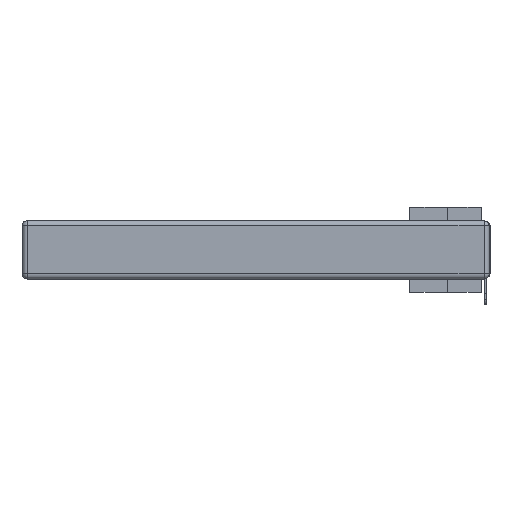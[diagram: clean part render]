
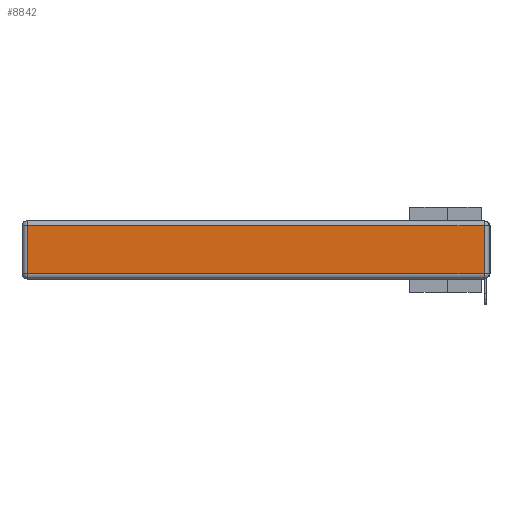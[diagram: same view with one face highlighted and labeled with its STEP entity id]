
A CAD part, left-side view. The second image highlights one B-rep face of the part: STEP entity #8842.
In plain terms, the highlighted planar face has unit normal (-1, 0, 0).
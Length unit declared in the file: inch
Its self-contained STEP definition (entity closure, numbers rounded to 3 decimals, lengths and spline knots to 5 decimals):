
#875 = CARTESIAN_POINT ( 'NONE',  ( 0., 2.75, -0.03 ) ) ;
#2345 = CARTESIAN_POINT ( 'NONE',  ( 0., 0.03, -0.03 ) ) ;
#2662 = DIRECTION ( 'NONE',  ( -1., 0., 0. ) ) ;
#2829 = CARTESIAN_POINT ( 'NONE',  ( 0., 0., -0.343 ) ) ;
#3519 = DIRECTION ( 'NONE',  ( 0., 1., 0. ) ) ;
#4431 = CARTESIAN_POINT ( 'NONE',  ( 0., 2.72, -0.343 ) ) ;
#6391 = EDGE_CURVE ( 'NONE', #31408, #27377, #11120, .T. ) ;
#7058 = ORIENTED_EDGE ( 'NONE', *, *, #6391, .T. ) ;
#8842 = ADVANCED_FACE ( 'NONE', ( #15121 ), #13142, .T. ) ;
#10361 = LINE ( 'NONE', #22984, #17152 ) ;
#10749 = VERTEX_POINT ( 'NONE', #23741 ) ;
#11120 = LINE ( 'NONE', #23893, #20728 ) ;
#11414 = EDGE_LOOP ( 'NONE', ( #19483, #7058, #20182, #12416 ) ) ;
#11934 = DIRECTION ( 'NONE',  ( 0., 0., -1. ) ) ;
#12416 = ORIENTED_EDGE ( 'NONE', *, *, #16696, .T. ) ;
#12655 = DIRECTION ( 'NONE',  ( 0., -1., 0. ) ) ;
#13142 = PLANE ( 'NONE',  #26629 ) ;
#13673 = LINE ( 'NONE', #875, #21818 ) ;
#15121 = FACE_OUTER_BOUND ( 'NONE', #11414, .T. ) ;
#16214 = DIRECTION ( 'NONE',  ( 0., 0., 1. ) ) ;
#16696 = EDGE_CURVE ( 'NONE', #23987, #10749, #16891, .T. ) ;
#16891 = LINE ( 'NONE', #4431, #18651 ) ;
#17152 = VECTOR ( 'NONE', #12655, 39.37008 ) ;
#17647 = EDGE_CURVE ( 'NONE', #10749, #31408, #10361, .T. ) ;
#18651 = VECTOR ( 'NONE', #11934, 39.37008 ) ;
#19483 = ORIENTED_EDGE ( 'NONE', *, *, #17647, .T. ) ;
#20182 = ORIENTED_EDGE ( 'NONE', *, *, #25946, .T. ) ;
#20728 = VECTOR ( 'NONE', #16214, 39.37008 ) ;
#20838 = DIRECTION ( 'NONE',  ( 0., 0., 1. ) ) ;
#21818 = VECTOR ( 'NONE', #3519, 39.37008 ) ;
#22749 = CARTESIAN_POINT ( 'NONE',  ( 0., 2.72, -0.03 ) ) ;
#22984 = CARTESIAN_POINT ( 'NONE',  ( 0., 0., -0.313 ) ) ;
#23741 = CARTESIAN_POINT ( 'NONE',  ( 0., 2.72, -0.313 ) ) ;
#23893 = CARTESIAN_POINT ( 'NONE',  ( 0., 0.03, -0.343 ) ) ;
#23987 = VERTEX_POINT ( 'NONE', #22749 ) ;
#25673 = CARTESIAN_POINT ( 'NONE',  ( 0., 0.03, -0.313 ) ) ;
#25946 = EDGE_CURVE ( 'NONE', #27377, #23987, #13673, .T. ) ;
#26629 = AXIS2_PLACEMENT_3D ( 'NONE', #2829, #2662, #20838 ) ;
#27377 = VERTEX_POINT ( 'NONE', #2345 ) ;
#31408 = VERTEX_POINT ( 'NONE', #25673 ) ;
